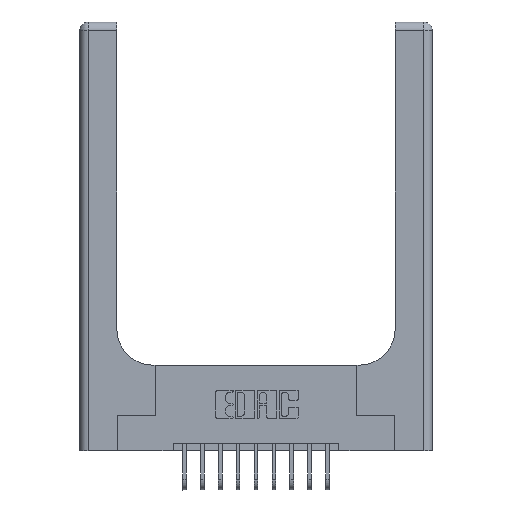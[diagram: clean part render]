
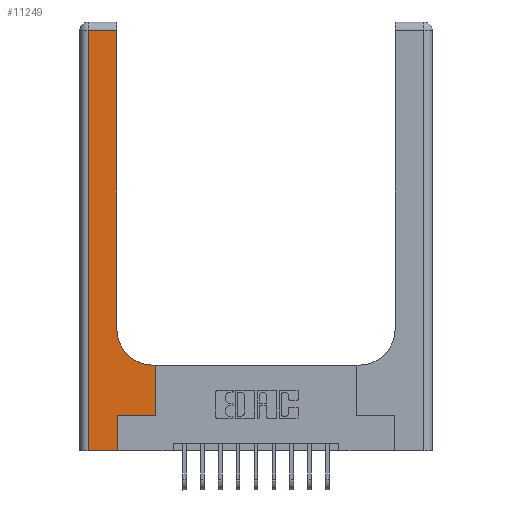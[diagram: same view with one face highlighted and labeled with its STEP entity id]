
A CAD part, top view. The second image highlights one B-rep face of the part: STEP entity #11249.
In plain terms, the highlighted planar face has unit normal (0, 0, 1).
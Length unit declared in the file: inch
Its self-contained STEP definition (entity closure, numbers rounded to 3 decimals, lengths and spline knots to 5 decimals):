
#450 = VECTOR ( 'NONE', #4447, 39.37008 ) ;
#464 = DIRECTION ( 'NONE',  ( 0., 1., 0. ) ) ;
#472 = VECTOR ( 'NONE', #464, 39.37008 ) ;
#735 = VECTOR ( 'NONE', #4720, 39.37008 ) ;
#999 = CARTESIAN_POINT ( 'NONE',  ( 0.26, 2.94, 0.37 ) ) ;
#1212 = VECTOR ( 'NONE', #9124, 39.37008 ) ;
#1497 = DIRECTION ( 'NONE',  ( -1., 0., 0. ) ) ;
#1531 = EDGE_LOOP ( 'NONE', ( #3692, #15301, #5144, #16412, #3170, #3618, #13056, #3238, #16976 ) ) ;
#1807 = CARTESIAN_POINT ( 'NONE',  ( 0.26, 0.85, 0.37 ) ) ;
#1968 = CARTESIAN_POINT ( 'NONE',  ( 0.528, 0.25, 0.37 ) ) ;
#3170 = ORIENTED_EDGE ( 'NONE', *, *, #8365, .T. ) ;
#3238 = ORIENTED_EDGE ( 'NONE', *, *, #5783, .T. ) ;
#3368 = VECTOR ( 'NONE', #8480, 39.37008 ) ;
#3463 = CARTESIAN_POINT ( 'NONE',  ( 0., 3., 0.37 ) ) ;
#3510 = PLANE ( 'NONE',  #6468 ) ;
#3618 = ORIENTED_EDGE ( 'NONE', *, *, #11690, .T. ) ;
#3692 = ORIENTED_EDGE ( 'NONE', *, *, #17306, .T. ) ;
#3810 = EDGE_CURVE ( 'NONE', #6206, #17205, #17074, .T. ) ;
#3995 = LINE ( 'NONE', #16118, #16929 ) ;
#4089 = VERTEX_POINT ( 'NONE', #11498 ) ;
#4447 = DIRECTION ( 'NONE',  ( 0., 1., 0. ) ) ;
#4513 = EDGE_CURVE ( 'NONE', #13207, #12701, #5951, .T. ) ;
#4720 = DIRECTION ( 'NONE',  ( 1., 0., 0. ) ) ;
#4788 = DIRECTION ( 'NONE',  ( -1., 0., 0. ) ) ;
#5014 = DIRECTION ( 'NONE',  ( 0., 0., -1. ) ) ;
#5144 = ORIENTED_EDGE ( 'NONE', *, *, #3810, .T. ) ;
#5146 = CARTESIAN_POINT ( 'NONE',  ( 0.265, 0.25, 0.37 ) ) ;
#5293 = LINE ( 'NONE', #10970, #472 ) ;
#5615 = DIRECTION ( 'NONE',  ( 0., -1., 0. ) ) ;
#5783 = EDGE_CURVE ( 'NONE', #9007, #13207, #3995, .T. ) ;
#5951 = CIRCLE ( 'NONE', #16533, 0.25 ) ;
#6206 = VERTEX_POINT ( 'NONE', #14253 ) ;
#6346 = DIRECTION ( 'NONE',  ( 0., 0., -1. ) ) ;
#6468 = AXIS2_PLACEMENT_3D ( 'NONE', #3463, #5014, #4788 ) ;
#6700 = DIRECTION ( 'NONE',  ( 1., 0., 0. ) ) ;
#7900 = VECTOR ( 'NONE', #6700, 39.37008 ) ;
#8365 = EDGE_CURVE ( 'NONE', #4089, #13667, #10667, .T. ) ;
#8377 = CARTESIAN_POINT ( 'NONE',  ( 0., 0., 0.37 ) ) ;
#8393 = CARTESIAN_POINT ( 'NONE',  ( 0.06, 3., 0.37 ) ) ;
#8480 = DIRECTION ( 'NONE',  ( 0., 1., 0. ) ) ;
#9007 = VERTEX_POINT ( 'NONE', #15846 ) ;
#9124 = DIRECTION ( 'NONE',  ( -1., 0., 0. ) ) ;
#9416 = LINE ( 'NONE', #1968, #450 ) ;
#10667 = LINE ( 'NONE', #11373, #3368 ) ;
#10970 = CARTESIAN_POINT ( 'NONE',  ( 0.26, 3., 0.37 ) ) ;
#11249 = ADVANCED_FACE ( 'NONE', ( #13953 ), #3510, .F. ) ;
#11373 = CARTESIAN_POINT ( 'NONE',  ( 0.265, 0., 0.37 ) ) ;
#11498 = CARTESIAN_POINT ( 'NONE',  ( 0.265, 0., 0.37 ) ) ;
#11551 = CARTESIAN_POINT ( 'NONE',  ( 0.528, 0.25, 0.37 ) ) ;
#11686 = EDGE_CURVE ( 'NONE', #14959, #6206, #13091, .T. ) ;
#11690 = EDGE_CURVE ( 'NONE', #13667, #15871, #16692, .T. ) ;
#12459 = VECTOR ( 'NONE', #5615, 39.37008 ) ;
#12701 = VERTEX_POINT ( 'NONE', #1807 ) ;
#13032 = LINE ( 'NONE', #8377, #735 ) ;
#13056 = ORIENTED_EDGE ( 'NONE', *, *, #15784, .T. ) ;
#13091 = LINE ( 'NONE', #13242, #1212 ) ;
#13207 = VERTEX_POINT ( 'NONE', #14832 ) ;
#13242 = CARTESIAN_POINT ( 'NONE',  ( 0., 2.94, 0.37 ) ) ;
#13330 = EDGE_CURVE ( 'NONE', #17205, #4089, #13032, .T. ) ;
#13667 = VERTEX_POINT ( 'NONE', #5146 ) ;
#13953 = FACE_OUTER_BOUND ( 'NONE', #1531, .T. ) ;
#14253 = CARTESIAN_POINT ( 'NONE',  ( 0.06, 2.94, 0.37 ) ) ;
#14322 = CARTESIAN_POINT ( 'NONE',  ( 0.51, 0.85, 0.37 ) ) ;
#14832 = CARTESIAN_POINT ( 'NONE',  ( 0.51, 0.6, 0.37 ) ) ;
#14959 = VERTEX_POINT ( 'NONE', #999 ) ;
#15301 = ORIENTED_EDGE ( 'NONE', *, *, #11686, .T. ) ;
#15703 = DIRECTION ( 'NONE',  ( 1., 0., 0. ) ) ;
#15784 = EDGE_CURVE ( 'NONE', #15871, #9007, #9416, .T. ) ;
#15846 = CARTESIAN_POINT ( 'NONE',  ( 0.528, 0.6, 0.37 ) ) ;
#15871 = VERTEX_POINT ( 'NONE', #11551 ) ;
#15989 = CARTESIAN_POINT ( 'NONE',  ( 0.265, 0.25, 0.37 ) ) ;
#16118 = CARTESIAN_POINT ( 'NONE',  ( 0.26, 0.6, 0.37 ) ) ;
#16242 = CARTESIAN_POINT ( 'NONE',  ( 0.06, 0., 0.37 ) ) ;
#16412 = ORIENTED_EDGE ( 'NONE', *, *, #13330, .T. ) ;
#16533 = AXIS2_PLACEMENT_3D ( 'NONE', #14322, #6346, #15703 ) ;
#16692 = LINE ( 'NONE', #15989, #7900 ) ;
#16929 = VECTOR ( 'NONE', #1497, 39.37008 ) ;
#16976 = ORIENTED_EDGE ( 'NONE', *, *, #4513, .T. ) ;
#17074 = LINE ( 'NONE', #8393, #12459 ) ;
#17205 = VERTEX_POINT ( 'NONE', #16242 ) ;
#17306 = EDGE_CURVE ( 'NONE', #12701, #14959, #5293, .T. ) ;
